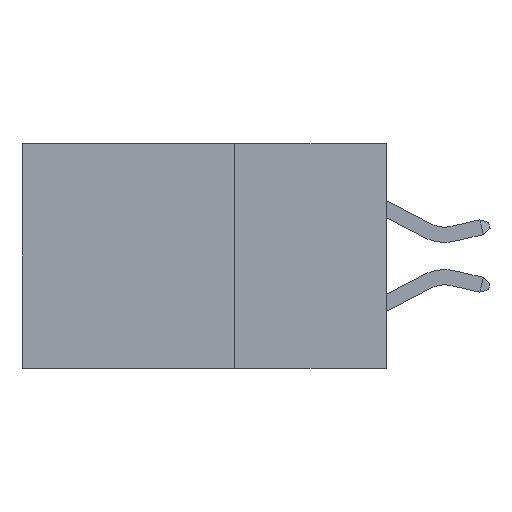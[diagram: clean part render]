
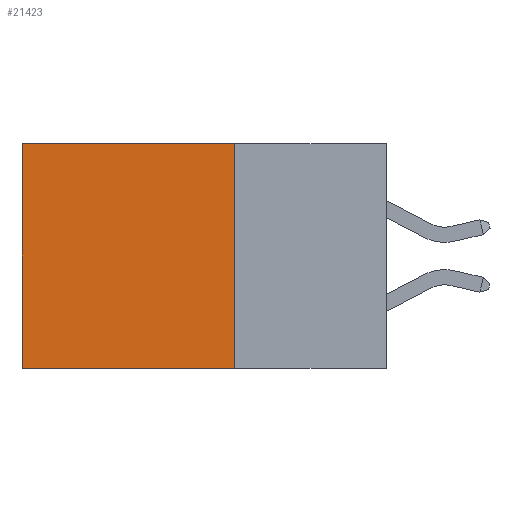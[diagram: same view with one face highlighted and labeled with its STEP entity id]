
A CAD part, left-side view. The second image highlights one B-rep face of the part: STEP entity #21423.
In plain terms, the highlighted planar face has unit normal (-1, 0, 0).
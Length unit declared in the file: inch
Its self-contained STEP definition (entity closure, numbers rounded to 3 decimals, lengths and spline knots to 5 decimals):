
#1171 = CARTESIAN_POINT ( 'NONE',  ( 0.298, 0.25, 0. ) ) ;
#1394 = DIRECTION ( 'NONE',  ( 1., 0., 0. ) ) ;
#2046 = EDGE_CURVE ( 'NONE', #11351, #6448, #6232, .T. ) ;
#2323 = ORIENTED_EDGE ( 'NONE', *, *, #2046, .F. ) ;
#3154 = ORIENTED_EDGE ( 'NONE', *, *, #4572, .F. ) ;
#3562 = FACE_OUTER_BOUND ( 'NONE', #21723, .T. ) ;
#4115 = EDGE_CURVE ( 'NONE', #15661, #6448, #16665, .T. ) ;
#4572 = EDGE_CURVE ( 'NONE', #19136, #11351, #20608, .T. ) ;
#5184 = VECTOR ( 'NONE', #13213, 39.37008 ) ;
#5668 = EDGE_CURVE ( 'NONE', #19136, #15661, #11061, .T. ) ;
#5779 = CARTESIAN_POINT ( 'NONE',  ( 0.298, 0.6, 0. ) ) ;
#5795 = CARTESIAN_POINT ( 'NONE',  ( 0.298, 0.25, 0. ) ) ;
#5866 = CARTESIAN_POINT ( 'NONE',  ( 0.298, 0.25, -0.37 ) ) ;
#6130 = VECTOR ( 'NONE', #16745, 39.37008 ) ;
#6232 = LINE ( 'NONE', #7341, #5184 ) ;
#6448 = VERTEX_POINT ( 'NONE', #21156 ) ;
#7341 = CARTESIAN_POINT ( 'NONE',  ( 0.298, 0.25, -0.37 ) ) ;
#8750 = DIRECTION ( 'NONE',  ( 0., 0., -1. ) ) ;
#9098 = AXIS2_PLACEMENT_3D ( 'NONE', #11377, #1394, #13057 ) ;
#10766 = ORIENTED_EDGE ( 'NONE', *, *, #5668, .T. ) ;
#11061 = LINE ( 'NONE', #1171, #6130 ) ;
#11351 = VERTEX_POINT ( 'NONE', #5866 ) ;
#11377 = CARTESIAN_POINT ( 'NONE',  ( 0.298, 0.25, 0. ) ) ;
#12724 = ORIENTED_EDGE ( 'NONE', *, *, #4115, .T. ) ;
#12896 = CARTESIAN_POINT ( 'NONE',  ( 0.298, 0.6, 0. ) ) ;
#12979 = PLANE ( 'NONE',  #9098 ) ;
#13057 = DIRECTION ( 'NONE',  ( 0., 0., -1. ) ) ;
#13213 = DIRECTION ( 'NONE',  ( 0., 1., 0. ) ) ;
#14320 = CARTESIAN_POINT ( 'NONE',  ( 0.298, 0.25, 0. ) ) ;
#15661 = VERTEX_POINT ( 'NONE', #5779 ) ;
#16113 = VECTOR ( 'NONE', #19159, 39.37008 ) ;
#16665 = LINE ( 'NONE', #12896, #21667 ) ;
#16745 = DIRECTION ( 'NONE',  ( 0., 1., 0. ) ) ;
#19136 = VERTEX_POINT ( 'NONE', #5795 ) ;
#19159 = DIRECTION ( 'NONE',  ( 0., 0., -1. ) ) ;
#20608 = LINE ( 'NONE', #14320, #16113 ) ;
#21156 = CARTESIAN_POINT ( 'NONE',  ( 0.298, 0.6, -0.37 ) ) ;
#21423 = ADVANCED_FACE ( 'NONE', ( #3562 ), #12979, .F. ) ;
#21667 = VECTOR ( 'NONE', #8750, 39.37008 ) ;
#21723 = EDGE_LOOP ( 'NONE', ( #12724, #2323, #3154, #10766 ) ) ;
